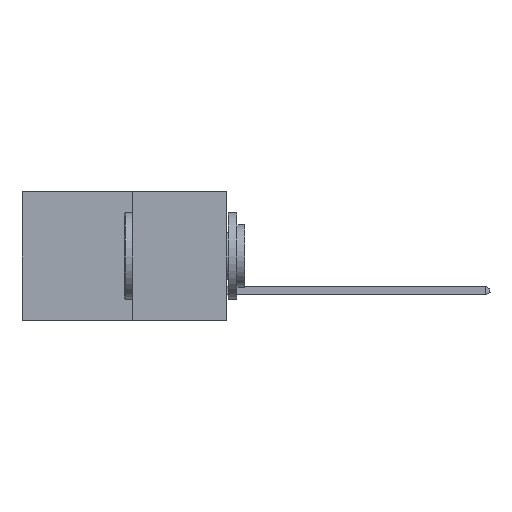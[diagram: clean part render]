
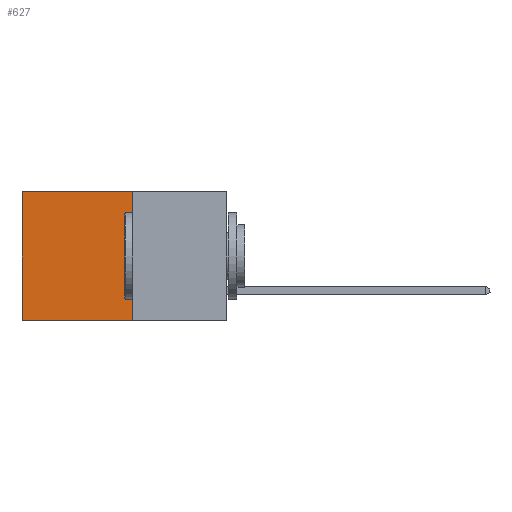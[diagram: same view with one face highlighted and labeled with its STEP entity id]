
A CAD part, left-side view. The second image highlights one B-rep face of the part: STEP entity #627.
In plain terms, the highlighted planar face has unit normal (-1, 0, 0).
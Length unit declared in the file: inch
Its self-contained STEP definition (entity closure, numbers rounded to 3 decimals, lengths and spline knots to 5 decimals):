
#627 = ADVANCED_FACE ( 'NONE', ( #7257 ), #8096, .F. ) ;
#1042 = EDGE_CURVE ( 'NONE', #9318, #2572, #1286, .T. ) ;
#1060 = VERTEX_POINT ( 'NONE', #3851 ) ;
#1286 = LINE ( 'NONE', #10742, #10684 ) ;
#2152 = DIRECTION ( 'NONE',  ( 0., 1., 0. ) ) ;
#2572 = VERTEX_POINT ( 'NONE', #10295 ) ;
#2712 = CARTESIAN_POINT ( 'NONE',  ( 0.277, 0.27, 0. ) ) ;
#2864 = VECTOR ( 'NONE', #13445, 39.37008 ) ;
#3301 = VECTOR ( 'NONE', #4220, 39.37008 ) ;
#3365 = DIRECTION ( 'NONE',  ( 0., 0., -1. ) ) ;
#3851 = CARTESIAN_POINT ( 'NONE',  ( 0.277, 0.59, 0. ) ) ;
#4172 = VECTOR ( 'NONE', #2152, 39.37008 ) ;
#4220 = DIRECTION ( 'NONE',  ( 0., 1., 0. ) ) ;
#4993 = EDGE_LOOP ( 'NONE', ( #14113, #5368, #12208, #6846 ) ) ;
#5368 = ORIENTED_EDGE ( 'NONE', *, *, #8287, .F. ) ;
#5470 = CARTESIAN_POINT ( 'NONE',  ( 0.277, 0.59, -0.37 ) ) ;
#5999 = VERTEX_POINT ( 'NONE', #8391 ) ;
#6846 = ORIENTED_EDGE ( 'NONE', *, *, #10145, .T. ) ;
#7257 = FACE_OUTER_BOUND ( 'NONE', #4993, .T. ) ;
#8069 = CARTESIAN_POINT ( 'NONE',  ( 0.277, 0.27, 0. ) ) ;
#8096 = PLANE ( 'NONE',  #13743 ) ;
#8287 = EDGE_CURVE ( 'NONE', #2572, #5999, #9554, .T. ) ;
#8391 = CARTESIAN_POINT ( 'NONE',  ( 0.277, 0.59, -0.37 ) ) ;
#8460 = DIRECTION ( 'NONE',  ( 1., 0., 0. ) ) ;
#8746 = LINE ( 'NONE', #5470, #2864 ) ;
#8784 = CARTESIAN_POINT ( 'NONE',  ( 0.277, 0.27, -0.37 ) ) ;
#9318 = VERTEX_POINT ( 'NONE', #2712 ) ;
#9554 = LINE ( 'NONE', #13356, #3301 ) ;
#10028 = EDGE_CURVE ( 'NONE', #1060, #5999, #8746, .T. ) ;
#10145 = EDGE_CURVE ( 'NONE', #9318, #1060, #13344, .T. ) ;
#10295 = CARTESIAN_POINT ( 'NONE',  ( 0.277, 0.27, -0.37 ) ) ;
#10684 = VECTOR ( 'NONE', #3365, 39.37008 ) ;
#10742 = CARTESIAN_POINT ( 'NONE',  ( 0.277, 0.27, -0.37 ) ) ;
#12208 = ORIENTED_EDGE ( 'NONE', *, *, #1042, .F. ) ;
#13344 = LINE ( 'NONE', #8069, #4172 ) ;
#13356 = CARTESIAN_POINT ( 'NONE',  ( 0.277, 0.27, -0.37 ) ) ;
#13445 = DIRECTION ( 'NONE',  ( 0., 0., -1. ) ) ;
#13743 = AXIS2_PLACEMENT_3D ( 'NONE', #8784, #8460, #14397 ) ;
#14113 = ORIENTED_EDGE ( 'NONE', *, *, #10028, .T. ) ;
#14397 = DIRECTION ( 'NONE',  ( 0., 0., -1. ) ) ;
